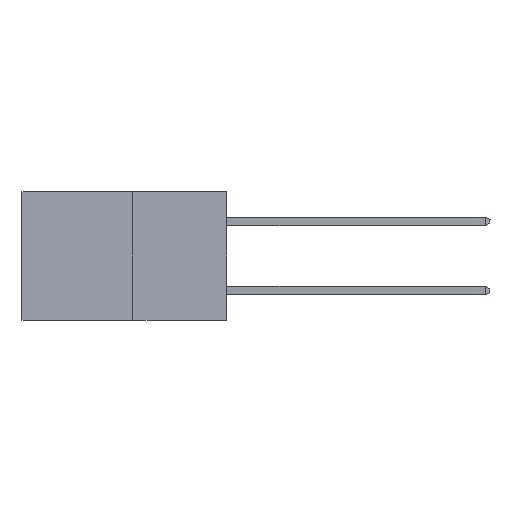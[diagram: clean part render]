
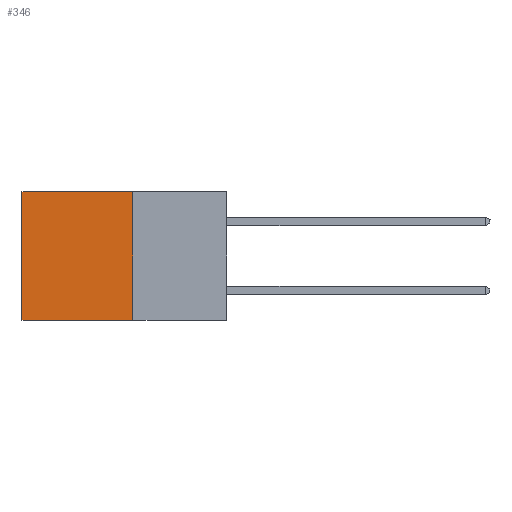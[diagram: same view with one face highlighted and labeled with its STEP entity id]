
A CAD part, left-side view. The second image highlights one B-rep face of the part: STEP entity #346.
In plain terms, the highlighted planar face has unit normal (-1, 0, 0).
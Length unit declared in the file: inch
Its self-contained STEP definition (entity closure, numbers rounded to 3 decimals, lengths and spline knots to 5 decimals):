
#279 = DIRECTION ( 'NONE',  ( 0., 0., -1. ) ) ;
#346 = ADVANCED_FACE ( 'NONE', ( #8100 ), #2746, .F. ) ;
#811 = ORIENTED_EDGE ( 'NONE', *, *, #7957, .T. ) ;
#962 = VECTOR ( 'NONE', #4811, 39.37008 ) ;
#1785 = EDGE_CURVE ( 'NONE', #5099, #3703, #4272, .T. ) ;
#1797 = DIRECTION ( 'NONE',  ( 1., 0., 0. ) ) ;
#1885 = LINE ( 'NONE', #8652, #7043 ) ;
#2028 = LINE ( 'NONE', #8710, #5384 ) ;
#2244 = LINE ( 'NONE', #5540, #3677 ) ;
#2506 = VERTEX_POINT ( 'NONE', #8438 ) ;
#2661 = EDGE_LOOP ( 'NONE', ( #811, #4560, #6312, #8047 ) ) ;
#2746 = PLANE ( 'NONE',  #4615 ) ;
#3677 = VECTOR ( 'NONE', #6221, 39.37008 ) ;
#3703 = VERTEX_POINT ( 'NONE', #6658 ) ;
#4132 = DIRECTION ( 'NONE',  ( 0., 1., 0. ) ) ;
#4272 = LINE ( 'NONE', #4964, #962 ) ;
#4476 = CARTESIAN_POINT ( 'NONE',  ( 0.277, 0.27, -0.37 ) ) ;
#4494 = CARTESIAN_POINT ( 'NONE',  ( 0.277, 0.59, -0.37 ) ) ;
#4560 = ORIENTED_EDGE ( 'NONE', *, *, #7808, .F. ) ;
#4615 = AXIS2_PLACEMENT_3D ( 'NONE', #4476, #1797, #279 ) ;
#4811 = DIRECTION ( 'NONE',  ( 0., 1., 0. ) ) ;
#4964 = CARTESIAN_POINT ( 'NONE',  ( 0.277, 0.27, 0. ) ) ;
#5099 = VERTEX_POINT ( 'NONE', #7122 ) ;
#5384 = VECTOR ( 'NONE', #6778, 39.37008 ) ;
#5540 = CARTESIAN_POINT ( 'NONE',  ( 0.277, 0.59, -0.37 ) ) ;
#5954 = VERTEX_POINT ( 'NONE', #4494 ) ;
#6221 = DIRECTION ( 'NONE',  ( 0., 0., -1. ) ) ;
#6312 = ORIENTED_EDGE ( 'NONE', *, *, #7026, .F. ) ;
#6658 = CARTESIAN_POINT ( 'NONE',  ( 0.277, 0.59, 0. ) ) ;
#6778 = DIRECTION ( 'NONE',  ( 0., 0., -1. ) ) ;
#7026 = EDGE_CURVE ( 'NONE', #5099, #2506, #2028, .T. ) ;
#7043 = VECTOR ( 'NONE', #4132, 39.37008 ) ;
#7122 = CARTESIAN_POINT ( 'NONE',  ( 0.277, 0.27, 0. ) ) ;
#7808 = EDGE_CURVE ( 'NONE', #2506, #5954, #1885, .T. ) ;
#7957 = EDGE_CURVE ( 'NONE', #3703, #5954, #2244, .T. ) ;
#8047 = ORIENTED_EDGE ( 'NONE', *, *, #1785, .T. ) ;
#8100 = FACE_OUTER_BOUND ( 'NONE', #2661, .T. ) ;
#8438 = CARTESIAN_POINT ( 'NONE',  ( 0.277, 0.27, -0.37 ) ) ;
#8652 = CARTESIAN_POINT ( 'NONE',  ( 0.277, 0.27, -0.37 ) ) ;
#8710 = CARTESIAN_POINT ( 'NONE',  ( 0.277, 0.27, -0.37 ) ) ;
